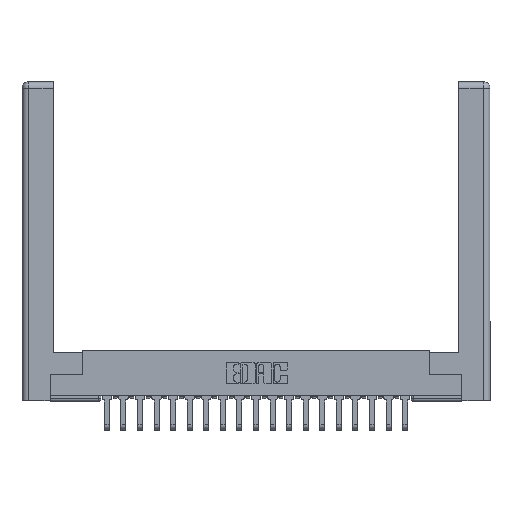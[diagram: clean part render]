
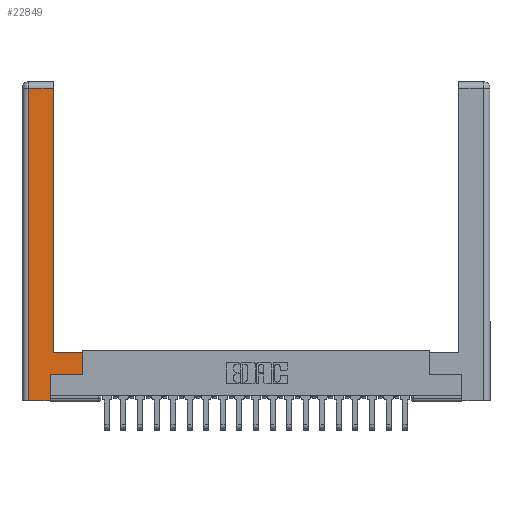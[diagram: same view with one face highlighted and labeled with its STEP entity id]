
A CAD part, top view. The second image highlights one B-rep face of the part: STEP entity #22849.
In plain terms, the highlighted planar face has unit normal (0, 0, 1).
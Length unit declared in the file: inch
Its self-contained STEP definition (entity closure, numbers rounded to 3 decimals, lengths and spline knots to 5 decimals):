
#422 = LINE ( 'NONE', #4572, #8484 ) ;
#799 = EDGE_CURVE ( 'NONE', #4693, #10556, #936, .T. ) ;
#901 = ORIENTED_EDGE ( 'NONE', *, *, #16926, .T. ) ;
#936 = LINE ( 'NONE', #7410, #19010 ) ;
#1053 = DIRECTION ( 'NONE',  ( 1., 0., 0. ) ) ;
#1643 = LINE ( 'NONE', #9515, #11423 ) ;
#1910 = ORIENTED_EDGE ( 'NONE', *, *, #799, .T. ) ;
#2281 = DIRECTION ( 'NONE',  ( -1., 0., 0. ) ) ;
#2452 = CARTESIAN_POINT ( 'NONE',  ( 0.265, 0., 0. ) ) ;
#2562 = VECTOR ( 'NONE', #17475, 39.37008 ) ;
#3614 = VECTOR ( 'NONE', #2281, 39.37008 ) ;
#3689 = EDGE_LOOP ( 'NONE', ( #21165, #17589, #12024, #901, #1910, #14899, #12828, #19471 ) ) ;
#3714 = VERTEX_POINT ( 'NONE', #23038 ) ;
#3951 = LINE ( 'NONE', #22133, #14568 ) ;
#3995 = DIRECTION ( 'NONE',  ( 0., -1., 0. ) ) ;
#4138 = DIRECTION ( 'NONE',  ( 0., 0., -1. ) ) ;
#4304 = VECTOR ( 'NONE', #3995, 39.37008 ) ;
#4572 = CARTESIAN_POINT ( 'NONE',  ( 0.565, 0.245, 0. ) ) ;
#4693 = VERTEX_POINT ( 'NONE', #7409 ) ;
#5990 = DIRECTION ( 'NONE',  ( -1., 0., 0. ) ) ;
#7228 = VERTEX_POINT ( 'NONE', #11417 ) ;
#7409 = CARTESIAN_POINT ( 'NONE',  ( 0.265, 0., 0. ) ) ;
#7410 = CARTESIAN_POINT ( 'NONE',  ( 0.265, 0.245, 0. ) ) ;
#7487 = DIRECTION ( 'NONE',  ( 0., 1., 0. ) ) ;
#7603 = DIRECTION ( 'NONE',  ( 0., 1., 0. ) ) ;
#8026 = LINE ( 'NONE', #12065, #2562 ) ;
#8484 = VECTOR ( 'NONE', #1053, 39.37008 ) ;
#9220 = CARTESIAN_POINT ( 'NONE',  ( 0.0615, 0., 0. ) ) ;
#9515 = CARTESIAN_POINT ( 'NONE',  ( 0.295, 3., 0. ) ) ;
#9745 = CARTESIAN_POINT ( 'NONE',  ( 0., 0., 0. ) ) ;
#9836 = EDGE_CURVE ( 'NONE', #15468, #16747, #12353, .T. ) ;
#10176 = EDGE_CURVE ( 'NONE', #7228, #15468, #8026, .T. ) ;
#10182 = LINE ( 'NONE', #18942, #3614 ) ;
#10556 = VERTEX_POINT ( 'NONE', #14349 ) ;
#11417 = CARTESIAN_POINT ( 'NONE',  ( 0.295, 2.94, 0. ) ) ;
#11423 = VECTOR ( 'NONE', #16483, 39.37008 ) ;
#12024 = ORIENTED_EDGE ( 'NONE', *, *, #9836, .T. ) ;
#12065 = CARTESIAN_POINT ( 'NONE',  ( 0.0615, 2.94, 0. ) ) ;
#12353 = LINE ( 'NONE', #22318, #4304 ) ;
#12828 = ORIENTED_EDGE ( 'NONE', *, *, #22753, .T. ) ;
#13178 = VERTEX_POINT ( 'NONE', #20070 ) ;
#14349 = CARTESIAN_POINT ( 'NONE',  ( 0.265, 0.245, 0. ) ) ;
#14568 = VECTOR ( 'NONE', #7603, 39.37008 ) ;
#14899 = ORIENTED_EDGE ( 'NONE', *, *, #20910, .T. ) ;
#15256 = DIRECTION ( 'NONE',  ( 1., 0., 0. ) ) ;
#15468 = VERTEX_POINT ( 'NONE', #23009 ) ;
#15649 = FACE_OUTER_BOUND ( 'NONE', #3689, .T. ) ;
#16483 = DIRECTION ( 'NONE',  ( 0., 1., 0. ) ) ;
#16747 = VERTEX_POINT ( 'NONE', #9220 ) ;
#16755 = CARTESIAN_POINT ( 'NONE',  ( 0.565, 0.45, 0. ) ) ;
#16926 = EDGE_CURVE ( 'NONE', #16747, #4693, #21311, .T. ) ;
#17475 = DIRECTION ( 'NONE',  ( -1., 0., 0. ) ) ;
#17589 = ORIENTED_EDGE ( 'NONE', *, *, #10176, .T. ) ;
#18116 = AXIS2_PLACEMENT_3D ( 'NONE', #9745, #4138, #5990 ) ;
#18942 = CARTESIAN_POINT ( 'NONE',  ( 0.295, 0.45, 0. ) ) ;
#19010 = VECTOR ( 'NONE', #7487, 39.37008 ) ;
#19342 = VERTEX_POINT ( 'NONE', #16755 ) ;
#19471 = ORIENTED_EDGE ( 'NONE', *, *, #20775, .T. ) ;
#20070 = CARTESIAN_POINT ( 'NONE',  ( 0.565, 0.245, 0. ) ) ;
#20171 = VECTOR ( 'NONE', #15256, 39.37008 ) ;
#20775 = EDGE_CURVE ( 'NONE', #19342, #3714, #10182, .T. ) ;
#20910 = EDGE_CURVE ( 'NONE', #10556, #13178, #422, .T. ) ;
#21165 = ORIENTED_EDGE ( 'NONE', *, *, #22685, .T. ) ;
#21311 = LINE ( 'NONE', #2452, #20171 ) ;
#22133 = CARTESIAN_POINT ( 'NONE',  ( 0.565, 0.45, 0. ) ) ;
#22318 = CARTESIAN_POINT ( 'NONE',  ( 0.0615, 0., 0. ) ) ;
#22677 = PLANE ( 'NONE',  #18116 ) ;
#22685 = EDGE_CURVE ( 'NONE', #3714, #7228, #1643, .T. ) ;
#22753 = EDGE_CURVE ( 'NONE', #13178, #19342, #3951, .T. ) ;
#22849 = ADVANCED_FACE ( 'NONE', ( #15649 ), #22677, .F. ) ;
#23009 = CARTESIAN_POINT ( 'NONE',  ( 0.0615, 2.94, 0. ) ) ;
#23038 = CARTESIAN_POINT ( 'NONE',  ( 0.295, 0.45, 0. ) ) ;
